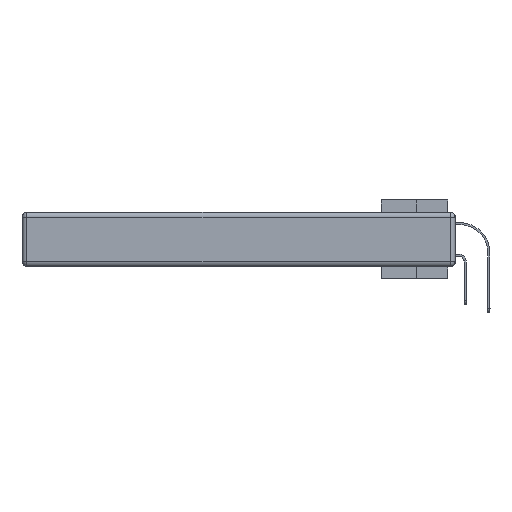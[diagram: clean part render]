
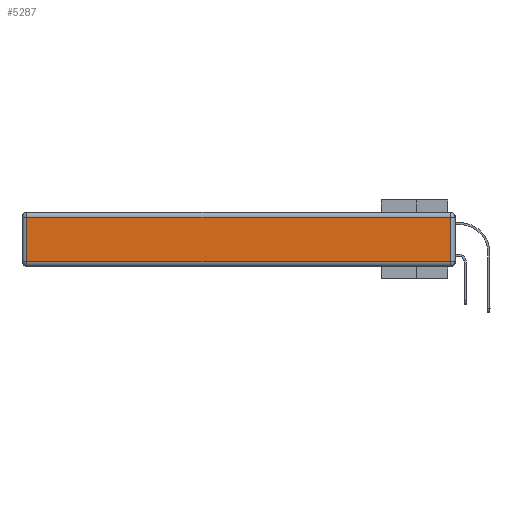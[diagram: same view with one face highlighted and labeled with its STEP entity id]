
A CAD part, left-side view. The second image highlights one B-rep face of the part: STEP entity #5287.
In plain terms, the highlighted planar face has unit normal (-1, 0, 0).
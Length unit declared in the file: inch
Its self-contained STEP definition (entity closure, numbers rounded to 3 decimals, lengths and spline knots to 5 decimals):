
#2490 = ORIENTED_EDGE ( 'NONE', *, *, #19841, .T. ) ;
#3207 = DIRECTION ( 'NONE',  ( 0., 0., 1. ) ) ;
#3447 = LINE ( 'NONE', #15359, #32555 ) ;
#4704 = CARTESIAN_POINT ( 'NONE',  ( 0., 0.03, -0.03 ) ) ;
#5287 = ADVANCED_FACE ( 'NONE', ( #23885 ), #35770, .T. ) ;
#5389 = DIRECTION ( 'NONE',  ( 0., 0., 1. ) ) ;
#5730 = EDGE_LOOP ( 'NONE', ( #8196, #19018, #34921, #2490 ) ) ;
#6635 = CARTESIAN_POINT ( 'NONE',  ( 0., 0., -0.313 ) ) ;
#8196 = ORIENTED_EDGE ( 'NONE', *, *, #31774, .T. ) ;
#9062 = CARTESIAN_POINT ( 'NONE',  ( 0., 0., -0.343 ) ) ;
#9559 = LINE ( 'NONE', #6635, #23918 ) ;
#9799 = CARTESIAN_POINT ( 'NONE',  ( 0., 0.03, -0.313 ) ) ;
#10324 = VERTEX_POINT ( 'NONE', #9799 ) ;
#11441 = CARTESIAN_POINT ( 'NONE',  ( 0., 0.03, -0.343 ) ) ;
#12113 = DIRECTION ( 'NONE',  ( 0., -1., 0. ) ) ;
#14779 = AXIS2_PLACEMENT_3D ( 'NONE', #9062, #29926, #3207 ) ;
#15359 = CARTESIAN_POINT ( 'NONE',  ( 0., 2.75, -0.03 ) ) ;
#16843 = LINE ( 'NONE', #34375, #22644 ) ;
#17799 = VERTEX_POINT ( 'NONE', #24657 ) ;
#17890 = DIRECTION ( 'NONE',  ( 0., 1., 0. ) ) ;
#19018 = ORIENTED_EDGE ( 'NONE', *, *, #29154, .T. ) ;
#19386 = DIRECTION ( 'NONE',  ( 0., 0., -1. ) ) ;
#19841 = EDGE_CURVE ( 'NONE', #17799, #33035, #16843, .T. ) ;
#19849 = LINE ( 'NONE', #11441, #23831 ) ;
#22644 = VECTOR ( 'NONE', #19386, 39.37008 ) ;
#23831 = VECTOR ( 'NONE', #5389, 39.37008 ) ;
#23885 = FACE_OUTER_BOUND ( 'NONE', #5730, .T. ) ;
#23918 = VECTOR ( 'NONE', #12113, 39.37008 ) ;
#24657 = CARTESIAN_POINT ( 'NONE',  ( 0., 2.72, -0.03 ) ) ;
#27192 = CARTESIAN_POINT ( 'NONE',  ( 0., 2.72, -0.313 ) ) ;
#29154 = EDGE_CURVE ( 'NONE', #10324, #30394, #19849, .T. ) ;
#29926 = DIRECTION ( 'NONE',  ( -1., 0., 0. ) ) ;
#30394 = VERTEX_POINT ( 'NONE', #4704 ) ;
#30703 = EDGE_CURVE ( 'NONE', #30394, #17799, #3447, .T. ) ;
#31774 = EDGE_CURVE ( 'NONE', #33035, #10324, #9559, .T. ) ;
#32555 = VECTOR ( 'NONE', #17890, 39.37008 ) ;
#33035 = VERTEX_POINT ( 'NONE', #27192 ) ;
#34375 = CARTESIAN_POINT ( 'NONE',  ( 0., 2.72, -0.343 ) ) ;
#34921 = ORIENTED_EDGE ( 'NONE', *, *, #30703, .T. ) ;
#35770 = PLANE ( 'NONE',  #14779 ) ;
